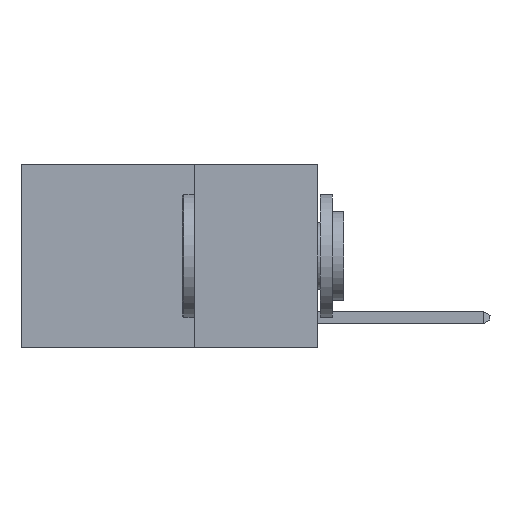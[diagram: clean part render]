
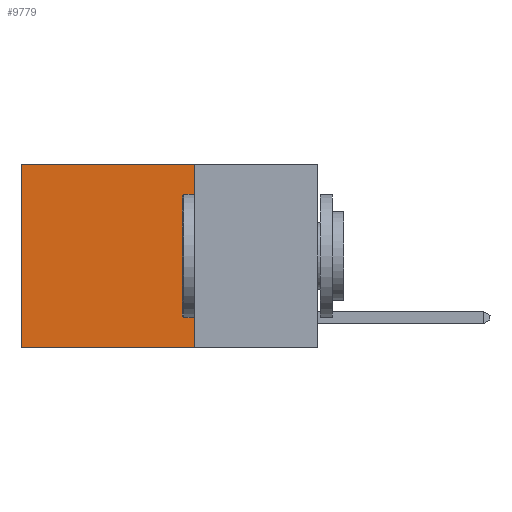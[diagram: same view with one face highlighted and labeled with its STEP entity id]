
A CAD part, left-side view. The second image highlights one B-rep face of the part: STEP entity #9779.
In plain terms, the highlighted planar face has unit normal (-1, 0, 0).
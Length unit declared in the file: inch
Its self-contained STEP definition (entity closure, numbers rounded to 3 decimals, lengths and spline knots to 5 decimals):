
#41 = DIRECTION ( 'NONE',  ( 0., 0., -1. ) ) ;
#1283 = VECTOR ( 'NONE', #10781, 39.37008 ) ;
#1401 = VECTOR ( 'NONE', #12744, 39.37008 ) ;
#1562 = CARTESIAN_POINT ( 'NONE',  ( 0.2625, 0.25, -0.37 ) ) ;
#2317 = ORIENTED_EDGE ( 'NONE', *, *, #5206, .T. ) ;
#3516 = AXIS2_PLACEMENT_3D ( 'NONE', #23991, #16705, #41 ) ;
#3724 = PLANE ( 'NONE',  #3516 ) ;
#5014 = EDGE_CURVE ( 'NONE', #8630, #22113, #7721, .T. ) ;
#5206 = EDGE_CURVE ( 'NONE', #6743, #6995, #6197, .T. ) ;
#5527 = LINE ( 'NONE', #18436, #1283 ) ;
#6197 = LINE ( 'NONE', #21463, #16618 ) ;
#6743 = VERTEX_POINT ( 'NONE', #14033 ) ;
#6995 = VERTEX_POINT ( 'NONE', #19717 ) ;
#7468 = CARTESIAN_POINT ( 'NONE',  ( 0.2625, 0.25, 0. ) ) ;
#7721 = LINE ( 'NONE', #14974, #10720 ) ;
#8630 = VERTEX_POINT ( 'NONE', #7468 ) ;
#9779 = ADVANCED_FACE ( 'NONE', ( #16832 ), #3724, .F. ) ;
#10204 = DIRECTION ( 'NONE',  ( 0., 0., -1. ) ) ;
#10246 = ORIENTED_EDGE ( 'NONE', *, *, #11306, .T. ) ;
#10720 = VECTOR ( 'NONE', #11166, 39.37008 ) ;
#10781 = DIRECTION ( 'NONE',  ( 0., 1., 0. ) ) ;
#11166 = DIRECTION ( 'NONE',  ( 0., 0., -1. ) ) ;
#11306 = EDGE_CURVE ( 'NONE', #8630, #6743, #5527, .T. ) ;
#12744 = DIRECTION ( 'NONE',  ( 0., 1., 0. ) ) ;
#14033 = CARTESIAN_POINT ( 'NONE',  ( 0.2625, 0.6, 0. ) ) ;
#14684 = LINE ( 'NONE', #1562, #1401 ) ;
#14974 = CARTESIAN_POINT ( 'NONE',  ( 0.2625, 0.25, 0. ) ) ;
#15043 = EDGE_CURVE ( 'NONE', #22113, #6995, #14684, .T. ) ;
#15537 = ORIENTED_EDGE ( 'NONE', *, *, #15043, .F. ) ;
#16618 = VECTOR ( 'NONE', #10204, 39.37008 ) ;
#16705 = DIRECTION ( 'NONE',  ( 1., 0., 0. ) ) ;
#16832 = FACE_OUTER_BOUND ( 'NONE', #20920, .T. ) ;
#18436 = CARTESIAN_POINT ( 'NONE',  ( 0.2625, 0.25, 0. ) ) ;
#19717 = CARTESIAN_POINT ( 'NONE',  ( 0.2625, 0.6, -0.37 ) ) ;
#20277 = CARTESIAN_POINT ( 'NONE',  ( 0.2625, 0.25, -0.37 ) ) ;
#20920 = EDGE_LOOP ( 'NONE', ( #2317, #15537, #22241, #10246 ) ) ;
#21463 = CARTESIAN_POINT ( 'NONE',  ( 0.2625, 0.6, 0. ) ) ;
#22113 = VERTEX_POINT ( 'NONE', #20277 ) ;
#22241 = ORIENTED_EDGE ( 'NONE', *, *, #5014, .F. ) ;
#23991 = CARTESIAN_POINT ( 'NONE',  ( 0.2625, 0.25, 0. ) ) ;
